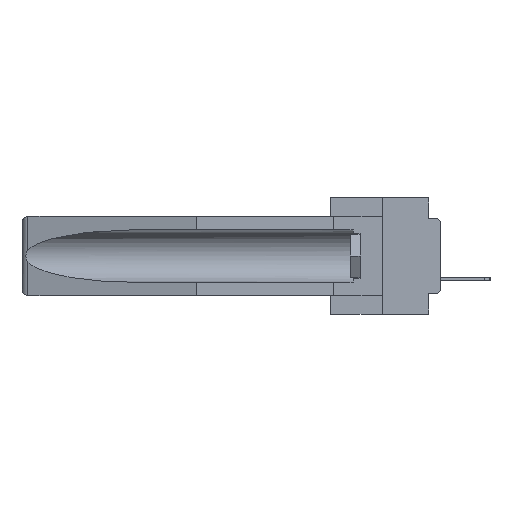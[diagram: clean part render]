
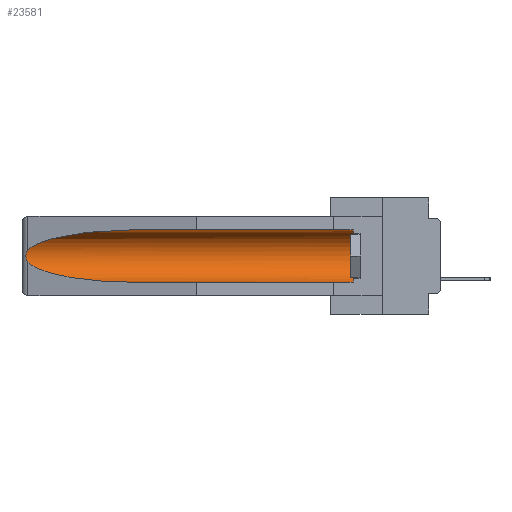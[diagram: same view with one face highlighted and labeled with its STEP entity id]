
A CAD part, left-side view. The second image highlights one B-rep face of the part: STEP entity #23581.
In plain terms, the highlighted cylindrical face has radius 2.857 mm (diameter 5.715 mm), a partial arc.
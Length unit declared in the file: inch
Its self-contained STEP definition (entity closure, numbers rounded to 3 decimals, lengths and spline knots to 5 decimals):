
#771 = CARTESIAN_POINT ( 'NONE',  ( 0.155, 1.07973, -0.284 ) ) ;
#891 = CYLINDRICAL_SURFACE ( 'NONE', #27184, 0.1125 ) ;
#1394 = EDGE_LOOP ( 'NONE', ( #8461, #1534, #20495, #17820, #13726, #25559 ) ) ;
#1534 = ORIENTED_EDGE ( 'NONE', *, *, #11429, .T. ) ;
#1945 = VERTEX_POINT ( 'NONE', #23184 ) ;
#4640 = CARTESIAN_POINT ( 'NONE',  ( 0.155, -0.30754, -0.059 ) ) ;
#5084 = CARTESIAN_POINT ( 'NONE',  ( 0.155, -0.30754, -0.284 ) ) ;
#5130 = VERTEX_POINT ( 'NONE', #22020 ) ;
#6690 = VERTEX_POINT ( 'NONE', #21370 ) ;
#6709 = CARTESIAN_POINT ( 'NONE',  ( 0.25451, 1.48313, -0.09465 ) ) ;
#7539 = VECTOR ( 'NONE', #17826, 39.37008 ) ;
#7752 = VECTOR ( 'NONE', #27073, 39.37008 ) ;
#8379 = EDGE_CURVE ( 'NONE', #6690, #1945, #28120, .T. ) ;
#8400 = CARTESIAN_POINT ( 'NONE',  ( 0.2673, 1.5327, -0.16383 ) ) ;
#8461 = ORIENTED_EDGE ( 'NONE', *, *, #8379, .T. ) ;
#8904 = AXIS2_PLACEMENT_3D ( 'NONE', #10515, #25822, #12716 ) ;
#9293 = EDGE_CURVE ( 'NONE', #17485, #24544, #28208, .T. ) ;
#9538 = CIRCLE ( 'NONE', #8904, 0.1125 ) ;
#10515 = CARTESIAN_POINT ( 'NONE',  ( 0.155, 0.126, -0.1715 ) ) ;
#10671 = CARTESIAN_POINT ( 'NONE',  ( 0.2675, 1.53308, -0.17534 ) ) ;
#11429 = EDGE_CURVE ( 'NONE', #1945, #17485, #15225, .T. ) ;
#12028 = CARTESIAN_POINT ( 'NONE',  ( 0.155, -0.30754, -0.1715 ) ) ;
#12475 = CARTESIAN_POINT ( 'NONE',  ( 0.155, 1.07973, -0.284 ) ) ;
#12716 = DIRECTION ( 'NONE',  ( 0., 0., 1. ) ) ;
#12843 = FACE_OUTER_BOUND ( 'NONE', #1394, .T. ) ;
#12857 = CARTESIAN_POINT ( 'NONE',  ( 0.26655, 1.53094, -0.18657 ) ) ;
#13074 = CARTESIAN_POINT ( 'NONE',  ( 0.155, 0.126, -0.059 ) ) ;
#13282 = CARTESIAN_POINT ( 'NONE',  ( 0.21114, 1.30732, -0.059 ) ) ;
#13726 = ORIENTED_EDGE ( 'NONE', *, *, #27014, .T. ) ;
#14188 = CARTESIAN_POINT ( 'NONE',  ( 0.26537, 1.52718, -0.19328 ) ) ;
#14198 = DIRECTION ( 'NONE',  ( 0., 1., 0. ) ) ;
#15034 = CARTESIAN_POINT ( 'NONE',  ( 0.26537, 1.52718, -0.19328 ) ) ;
#15225 = B_SPLINE_CURVE_WITH_KNOTS ( 'NONE', 3,
 ( #19327, #17119, #21557, #8400, #23777, #10671, #25973, #12857, #28104, #15034 ),
 .UNSPECIFIED., .F., .F.,
 ( 4, 2, 2, 2, 4 ),
 ( 0., 0.00029, 0.00058, 0.00087, 0.00117 ),
 .UNSPECIFIED. ) ;
#16995 = CARTESIAN_POINT ( 'NONE',  ( 0.26537, 1.52718, -0.19328 ) ) ;
#17119 = CARTESIAN_POINT ( 'NONE',  ( 0.26597, 1.52961, -0.15275 ) ) ;
#17485 = VERTEX_POINT ( 'NONE', #16995 ) ;
#17820 = ORIENTED_EDGE ( 'NONE', *, *, #27245, .F. ) ;
#17826 = DIRECTION ( 'NONE',  ( 0., 1., 0. ) ) ;
#19327 = CARTESIAN_POINT ( 'NONE',  ( 0.26537, 1.52718, -0.14972 ) ) ;
#19423 = LINE ( 'NONE', #5084, #7752 ) ;
#20495 = ORIENTED_EDGE ( 'NONE', *, *, #9293, .T. ) ;
#21370 = CARTESIAN_POINT ( 'NONE',  ( 0.155, 1.07973, -0.059 ) ) ;
#21557 = CARTESIAN_POINT ( 'NONE',  ( 0.26654, 1.53092, -0.15636 ) ) ;
#22020 = CARTESIAN_POINT ( 'NONE',  ( 0.155, 0.126, -0.284 ) ) ;
#22065 = CARTESIAN_POINT ( 'NONE',  ( 0.26537, 1.52718, -0.14972 ) ) ;
#22908 = CARTESIAN_POINT ( 'NONE',  ( 0.25451, 1.48313, -0.24835 ) ) ;
#22924 = DIRECTION ( 'NONE',  ( 0., 0., 1. ) ) ;
#23016 = LINE ( 'NONE', #4640, #7539 ) ;
#23184 = CARTESIAN_POINT ( 'NONE',  ( 0.26537, 1.52718, -0.14972 ) ) ;
#23279 = VERTEX_POINT ( 'NONE', #13074 ) ;
#23581 = ADVANCED_FACE ( 'NONE', ( #12843 ), #891, .F. ) ;
#23777 = CARTESIAN_POINT ( 'NONE',  ( 0.2675, 1.53308, -0.16763 ) ) ;
#24544 = VERTEX_POINT ( 'NONE', #12475 ) ;
#25121 = CARTESIAN_POINT ( 'NONE',  ( 0.21114, 1.30732, -0.284 ) ) ;
#25360 = EDGE_CURVE ( 'NONE', #23279, #6690, #23016, .T. ) ;
#25559 = ORIENTED_EDGE ( 'NONE', *, *, #25360, .T. ) ;
#25822 = DIRECTION ( 'NONE',  ( 0., -1., 0. ) ) ;
#25973 = CARTESIAN_POINT ( 'NONE',  ( 0.2673, 1.53269, -0.17917 ) ) ;
#27014 = EDGE_CURVE ( 'NONE', #5130, #23279, #9538, .T. ) ;
#27073 = DIRECTION ( 'NONE',  ( 0., 1., 0. ) ) ;
#27184 = AXIS2_PLACEMENT_3D ( 'NONE', #12028, #14198, #22924 ) ;
#27245 = EDGE_CURVE ( 'NONE', #5130, #24544, #19423, .T. ) ;
#28104 = CARTESIAN_POINT ( 'NONE',  ( 0.26597, 1.5296, -0.19026 ) ) ;
#28120 =( BOUNDED_CURVE ( )  B_SPLINE_CURVE ( 3, ( #28511, #13282, #6709, #22065 ),
 .UNSPECIFIED., .F., .F. ) 
 B_SPLINE_CURVE_WITH_KNOTS ( ( 4, 4 ),
 ( 4.71239, 6.08839 ),
 .UNSPECIFIED. ) 
 CURVE ( )  GEOMETRIC_REPRESENTATION_ITEM ( )  RATIONAL_B_SPLINE_CURVE ( ( 1., 0.848, 0.848, 1. ) ) 
 REPRESENTATION_ITEM ( '' )  );
#28208 =( BOUNDED_CURVE ( )  B_SPLINE_CURVE ( 3, ( #14188, #22908, #25121, #771 ),
 .UNSPECIFIED., .F., .F. ) 
 B_SPLINE_CURVE_WITH_KNOTS ( ( 4, 4 ),
 ( 0.1948, 1.5708 ),
 .UNSPECIFIED. ) 
 CURVE ( )  GEOMETRIC_REPRESENTATION_ITEM ( )  RATIONAL_B_SPLINE_CURVE ( ( 1., 0.848, 0.848, 1. ) ) 
 REPRESENTATION_ITEM ( '' )  );
#28511 = CARTESIAN_POINT ( 'NONE',  ( 0.155, 1.07973, -0.059 ) ) ;
